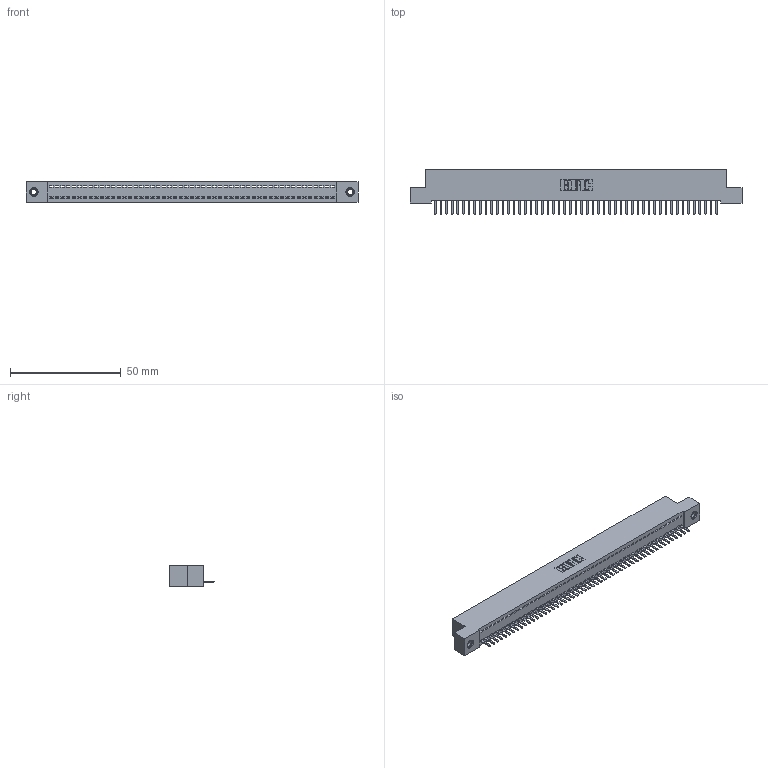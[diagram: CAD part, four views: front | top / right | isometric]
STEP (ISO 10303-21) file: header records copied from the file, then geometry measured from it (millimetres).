
FILE_DESCRIPTION (( 'STEP AP203' ), '1' );
FILE_NAME ('392-051-520-107.STEP', '2019-10-08T11:50:09', ( '' ), ( '' ), 'SwSTEP 2.0', 'SolidWorks 2016', '' );
FILE_SCHEMA (( 'CONFIG_CONTROL_DESIGN' ));
Length unit declared in the file: inch
Products named in the file (4): 342 Part_TI; 345-292-001_345-293-120; 345-250-001_345-250-005-103; 392-051-520-107
Assembly tree (54 placements, depth 2):
  392-051-520-107
    342 Part_TI
    345-292-001_345-293-120  x51
    345-250-001_345-250-005-103  x2
Bounding box: 149.86 x 20.02 x 9.4 mm (x, y, z)
Volume: 13013.5 mm3; surface area: 18840.8 mm2
Topology: 54 solids, 54 shells, 3332 faces, 9819 edges, 6402 vertices
Faces by surface type: plane 2342, cylinder 974, cone 12, torus 4
Entity records: 31182 total; most frequent: CARTESIAN_POINT 5370, ORIENTED_EDGE 5338, DIRECTION 4533, EDGE_CURVE 2669, LINE 2517, VECTOR 2517, VERTEX_POINT 1772, AXIS2_PLACEMENT_3D 1008
